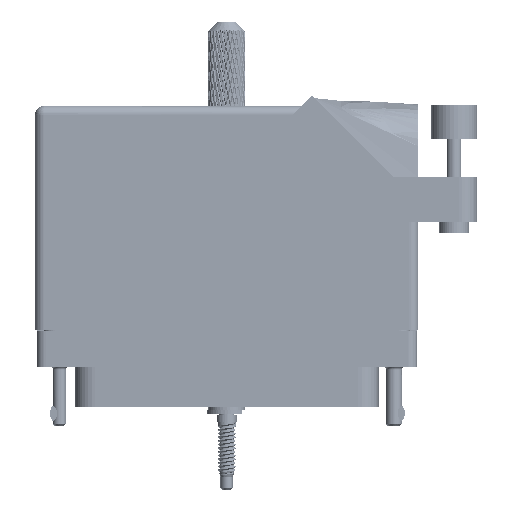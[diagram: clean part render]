
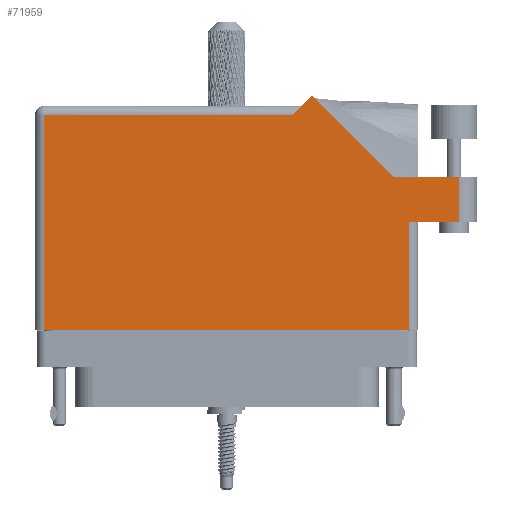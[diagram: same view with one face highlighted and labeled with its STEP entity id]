
A CAD part, front view. The second image highlights one B-rep face of the part: STEP entity #71959.
In plain terms, the highlighted face is planar.
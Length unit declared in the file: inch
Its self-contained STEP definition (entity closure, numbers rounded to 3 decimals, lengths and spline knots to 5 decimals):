
#769 = CARTESIAN_POINT ( 'NONE',  ( 1.244, 0.637, 0.455 ) ) ;
#1667 = CARTESIAN_POINT ( 'NONE',  ( 0.513, 1.43, 0.455 ) ) ;
#5154 = DIRECTION ( 'NONE',  ( -1., 0., 0. ) ) ;
#9247 = VERTEX_POINT ( 'NONE', #57504 ) ;
#9664 = DIRECTION ( 'NONE',  ( -0.707, 0.707, 0. ) ) ;
#14427 = VERTEX_POINT ( 'NONE', #85298 ) ;
#18080 = EDGE_CURVE ( 'NONE', #77168, #115542, #33104, .T. ) ;
#19110 = VECTOR ( 'NONE', #92165, 39.37008 ) ;
#19472 = LINE ( 'NONE', #59285, #21871 ) ;
#21486 = LINE ( 'NONE', #1667, #89549 ) ;
#21871 = VECTOR ( 'NONE', #108744, 39.37008 ) ;
#22747 = CARTESIAN_POINT ( 'NONE',  ( -1.244, -0.1, 0.455 ) ) ;
#31425 = ORIENTED_EDGE ( 'NONE', *, *, #91685, .T. ) ;
#31962 = CARTESIAN_POINT ( 'NONE',  ( 1.581, 0.944, 0.455 ) ) ;
#32046 = VECTOR ( 'NONE', #9664, 39.37008 ) ;
#33104 = LINE ( 'NONE', #101813, #19110 ) ;
#36334 = EDGE_CURVE ( 'NONE', #9247, #41355, #68133, .T. ) ;
#36616 = EDGE_CURVE ( 'NONE', #116142, #9247, #54537, .T. ) ;
#36803 = EDGE_CURVE ( 'NONE', #115542, #118841, #101326, .T. ) ;
#37323 = CARTESIAN_POINT ( 'NONE',  ( -1.244, -0.1, 0.455 ) ) ;
#38944 = EDGE_CURVE ( 'NONE', #97463, #14427, #78938, .T. ) ;
#41355 = VERTEX_POINT ( 'NONE', #22747 ) ;
#42256 = CARTESIAN_POINT ( 'NONE',  ( 0.451, 1.368, 0.455 ) ) ;
#44500 = EDGE_LOOP ( 'NONE', ( #49071, #77982, #113264, #93876, #125330, #71876, #116846, #31425, #76499 ) ) ;
#49071 = ORIENTED_EDGE ( 'NONE', *, *, #18080, .T. ) ;
#50947 = AXIS2_PLACEMENT_3D ( 'NONE', #53082, #52461, #92242 ) ;
#52461 = DIRECTION ( 'NONE',  ( 0., 0., -1. ) ) ;
#53082 = CARTESIAN_POINT ( 'NONE',  ( -1.306, 1.43, 0.455 ) ) ;
#54517 = CARTESIAN_POINT ( 'NONE',  ( 1.244, 0.637, 0.455 ) ) ;
#54537 = LINE ( 'NONE', #85320, #107767 ) ;
#57504 = CARTESIAN_POINT ( 'NONE',  ( -1.244, 1.368, 0.455 ) ) ;
#59285 = CARTESIAN_POINT ( 'NONE',  ( 1.706, 0.944, 0.455 ) ) ;
#60470 = VECTOR ( 'NONE', #97033, 39.37008 ) ;
#60822 = FACE_OUTER_BOUND ( 'NONE', #44500, .T. ) ;
#68133 = LINE ( 'NONE', #37323, #60470 ) ;
#68158 = DIRECTION ( 'NONE',  ( 0., 1., 0. ) ) ;
#69400 = CARTESIAN_POINT ( 'NONE',  ( 1.244, -0.1, 0.455 ) ) ;
#71555 = DIRECTION ( 'NONE',  ( -0.707, -0.707, 0. ) ) ;
#71876 = ORIENTED_EDGE ( 'NONE', *, *, #36616, .T. ) ;
#71959 = ADVANCED_FACE ( 'NONE', ( #60822 ), #72338, .F. ) ;
#72338 = PLANE ( 'NONE',  #50947 ) ;
#76499 = ORIENTED_EDGE ( 'NONE', *, *, #101174, .T. ) ;
#77168 = VERTEX_POINT ( 'NONE', #54517 ) ;
#77982 = ORIENTED_EDGE ( 'NONE', *, *, #36803, .T. ) ;
#78938 = LINE ( 'NONE', #87318, #32046 ) ;
#82799 = VERTEX_POINT ( 'NONE', #69400 ) ;
#85298 = CARTESIAN_POINT ( 'NONE',  ( 0.58371, 1.50071, 0.455 ) ) ;
#85320 = CARTESIAN_POINT ( 'NONE',  ( -1.306, 1.368, 0.455 ) ) ;
#86703 = EDGE_CURVE ( 'NONE', #118841, #97463, #19472, .T. ) ;
#87318 = CARTESIAN_POINT ( 'NONE',  ( 1.14042, 0.944, 0.455 ) ) ;
#88031 = LINE ( 'NONE', #769, #107105 ) ;
#88870 = LINE ( 'NONE', #91405, #94104 ) ;
#89107 = CARTESIAN_POINT ( 'NONE',  ( 1.581, 0.944, 0.455 ) ) ;
#89549 = VECTOR ( 'NONE', #71555, 39.37008 ) ;
#91405 = CARTESIAN_POINT ( 'NONE',  ( -1.306, -0.1, 0.455 ) ) ;
#91685 = EDGE_CURVE ( 'NONE', #41355, #82799, #88870, .T. ) ;
#92165 = DIRECTION ( 'NONE',  ( 1., 0., 0. ) ) ;
#92242 = DIRECTION ( 'NONE',  ( -1., 0., 0. ) ) ;
#93876 = ORIENTED_EDGE ( 'NONE', *, *, #38944, .T. ) ;
#94104 = VECTOR ( 'NONE', #108152, 39.37008 ) ;
#97033 = DIRECTION ( 'NONE',  ( 0., -1., 0. ) ) ;
#97463 = VERTEX_POINT ( 'NONE', #104278 ) ;
#101174 = EDGE_CURVE ( 'NONE', #82799, #77168, #88031, .T. ) ;
#101326 = LINE ( 'NONE', #31962, #124171 ) ;
#101813 = CARTESIAN_POINT ( 'NONE',  ( 1.306, 0.637, 0.455 ) ) ;
#104278 = CARTESIAN_POINT ( 'NONE',  ( 1.14042, 0.944, 0.455 ) ) ;
#107105 = VECTOR ( 'NONE', #68158, 39.37008 ) ;
#107767 = VECTOR ( 'NONE', #5154, 39.37008 ) ;
#108152 = DIRECTION ( 'NONE',  ( 1., 0., 0. ) ) ;
#108744 = DIRECTION ( 'NONE',  ( -1., 0., 0. ) ) ;
#110334 = DIRECTION ( 'NONE',  ( 0., 1., 0. ) ) ;
#112089 = EDGE_CURVE ( 'NONE', #14427, #116142, #21486, .T. ) ;
#113264 = ORIENTED_EDGE ( 'NONE', *, *, #86703, .T. ) ;
#115542 = VERTEX_POINT ( 'NONE', #118842 ) ;
#116142 = VERTEX_POINT ( 'NONE', #42256 ) ;
#116846 = ORIENTED_EDGE ( 'NONE', *, *, #36334, .T. ) ;
#118841 = VERTEX_POINT ( 'NONE', #89107 ) ;
#118842 = CARTESIAN_POINT ( 'NONE',  ( 1.581, 0.637, 0.455 ) ) ;
#124171 = VECTOR ( 'NONE', #110334, 39.37008 ) ;
#125330 = ORIENTED_EDGE ( 'NONE', *, *, #112089, .T. ) ;
